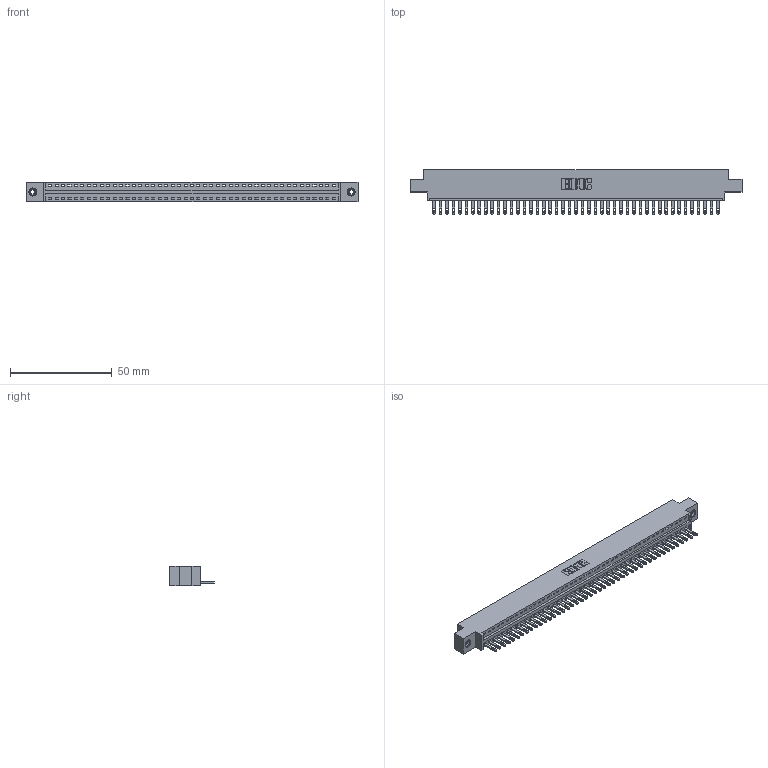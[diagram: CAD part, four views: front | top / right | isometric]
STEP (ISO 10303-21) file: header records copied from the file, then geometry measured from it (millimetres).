
FILE_DESCRIPTION (( 'STEP AP203' ), '1' );
FILE_NAME ('346-045-500-608.STEP', '2022-05-09T17:58:19', ( '' ), ( '' ), 'SwSTEP 2.0', 'SolidWorks 2020', '' );
FILE_SCHEMA (( 'CONFIG_CONTROL_DESIGN' ));
Length unit declared in the file: inch
Products named in the file (4): 346 Part_0.170 Offset - 0.156 Dia-TI; 345-250-001_345-250-003-102; 345-292-001_345-293-100; 346-045-500-608
Assembly tree (48 placements, depth 2):
  346-045-500-608
    346 Part_0.170 Offset - 0.156 Dia-TI
    345-292-001_345-293-100  x45
    345-250-001_345-250-003-102  x2
Bounding box: 163.45 x 21.84 x 9.4 mm (x, y, z)
Volume: 15533.1 mm3; surface area: 19733.7 mm2
Topology: 48 solids, 48 shells, 2616 faces, 8037 edges, 5350 vertices
Faces by surface type: plane 1642, cylinder 958, cone 12, torus 4
Entity records: 28772 total; most frequent: CARTESIAN_POINT 4914, ORIENTED_EDGE 4886, DIRECTION 4359, EDGE_CURVE 2443, LINE 2107, VECTOR 2107, VERTEX_POINT 1624, AXIS2_PLACEMENT_3D 1126
